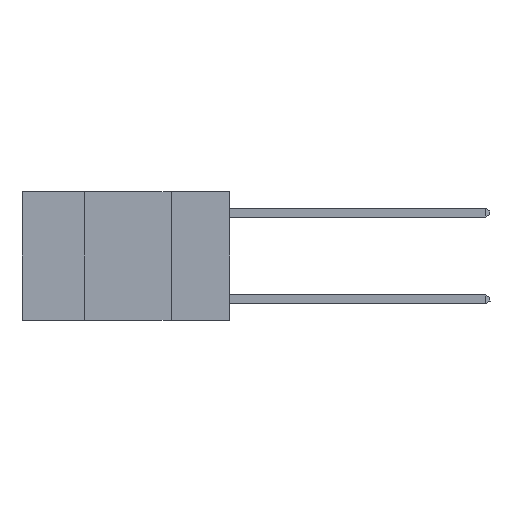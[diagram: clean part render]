
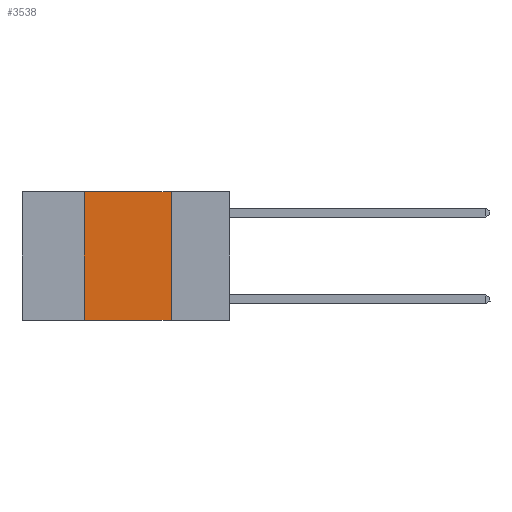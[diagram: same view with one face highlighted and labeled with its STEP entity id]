
A CAD part, left-side view. The second image highlights one B-rep face of the part: STEP entity #3538.
In plain terms, the highlighted planar face has unit normal (-1, 0, 0).
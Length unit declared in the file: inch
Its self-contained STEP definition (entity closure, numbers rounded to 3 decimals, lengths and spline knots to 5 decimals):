
#222 = CARTESIAN_POINT ( 'NONE',  ( 0., 0.17, -0.37 ) ) ;
#608 = CARTESIAN_POINT ( 'NONE',  ( 0., 0.42, 0. ) ) ;
#877 = ORIENTED_EDGE ( 'NONE', *, *, #9846, .F. ) ;
#914 = CARTESIAN_POINT ( 'NONE',  ( 0., 0.6, 0. ) ) ;
#942 = ORIENTED_EDGE ( 'NONE', *, *, #11545, .F. ) ;
#1014 = ORIENTED_EDGE ( 'NONE', *, *, #8526, .F. ) ;
#1053 = ORIENTED_EDGE ( 'NONE', *, *, #7912, .T. ) ;
#1076 = VERTEX_POINT ( 'NONE', #608 ) ;
#1377 = CARTESIAN_POINT ( 'NONE',  ( 0., 0.6, -0.37 ) ) ;
#1888 = DIRECTION ( 'NONE',  ( 0., -1., 0. ) ) ;
#3001 = DIRECTION ( 'NONE',  ( 1., 0., 0. ) ) ;
#3538 = ADVANCED_FACE ( 'NONE', ( #4236 ), #4935, .F. ) ;
#3607 = VECTOR ( 'NONE', #5466, 39.37008 ) ;
#3839 = LINE ( 'NONE', #3893, #8673 ) ;
#3893 = CARTESIAN_POINT ( 'NONE',  ( 0., 0.6, 0. ) ) ;
#4236 = FACE_OUTER_BOUND ( 'NONE', #11322, .T. ) ;
#4276 = VECTOR ( 'NONE', #10814, 39.37008 ) ;
#4353 = VERTEX_POINT ( 'NONE', #11957 ) ;
#4935 = PLANE ( 'NONE',  #12550 ) ;
#5466 = DIRECTION ( 'NONE',  ( 0., 0., 1. ) ) ;
#7410 = VERTEX_POINT ( 'NONE', #222 ) ;
#7912 = EDGE_CURVE ( 'NONE', #11963, #7410, #11968, .T. ) ;
#8403 = CARTESIAN_POINT ( 'NONE',  ( 0., 0.42, -0.37 ) ) ;
#8526 = EDGE_CURVE ( 'NONE', #11963, #1076, #11617, .T. ) ;
#8673 = VECTOR ( 'NONE', #1888, 39.37008 ) ;
#9328 = VECTOR ( 'NONE', #10435, 39.37008 ) ;
#9453 = CARTESIAN_POINT ( 'NONE',  ( 0., 0.17, 0. ) ) ;
#9815 = DIRECTION ( 'NONE',  ( 0., 0., -1. ) ) ;
#9846 = EDGE_CURVE ( 'NONE', #4353, #7410, #12172, .T. ) ;
#10435 = DIRECTION ( 'NONE',  ( 0., 0., -1. ) ) ;
#10814 = DIRECTION ( 'NONE',  ( 0., -1., 0. ) ) ;
#11246 = CARTESIAN_POINT ( 'NONE',  ( 0., 0.42, 0. ) ) ;
#11322 = EDGE_LOOP ( 'NONE', ( #877, #942, #1014, #1053 ) ) ;
#11545 = EDGE_CURVE ( 'NONE', #1076, #4353, #3839, .T. ) ;
#11617 = LINE ( 'NONE', #11246, #3607 ) ;
#11957 = CARTESIAN_POINT ( 'NONE',  ( 0., 0.17, 0. ) ) ;
#11963 = VERTEX_POINT ( 'NONE', #8403 ) ;
#11968 = LINE ( 'NONE', #1377, #4276 ) ;
#12172 = LINE ( 'NONE', #9453, #9328 ) ;
#12550 = AXIS2_PLACEMENT_3D ( 'NONE', #914, #3001, #9815 ) ;
